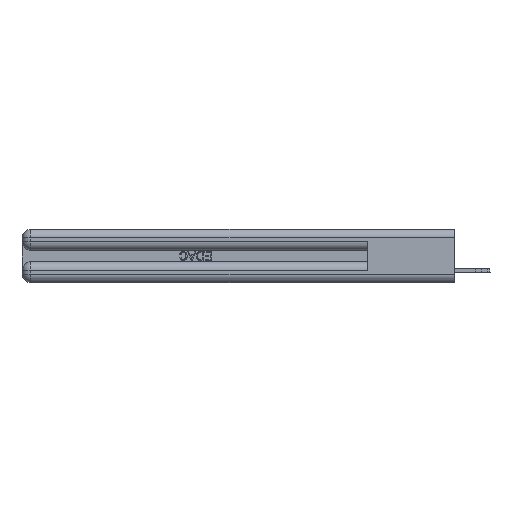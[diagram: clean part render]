
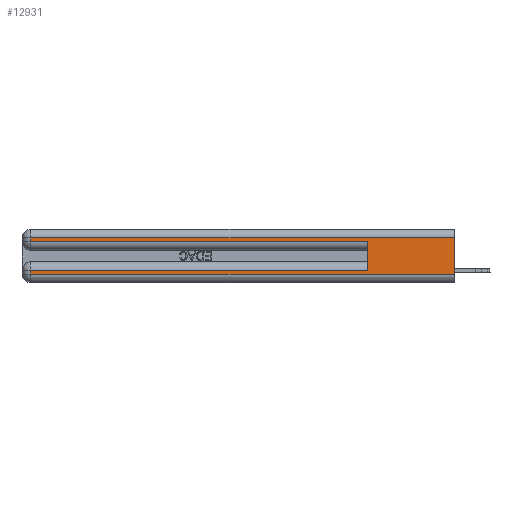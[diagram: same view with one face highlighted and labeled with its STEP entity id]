
A CAD part, left-side view. The second image highlights one B-rep face of the part: STEP entity #12931.
In plain terms, the highlighted planar face has unit normal (-1, 0, 0).
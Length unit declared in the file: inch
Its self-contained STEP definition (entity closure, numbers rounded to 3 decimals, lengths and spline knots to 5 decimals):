
#27 = EDGE_LOOP ( 'NONE', ( #20840, #12368, #30266, #17095, #7942, #33751, #11199, #32306 ) ) ;
#104 = LINE ( 'NONE', #30512, #34752 ) ;
#208 = EDGE_CURVE ( 'NONE', #19348, #15938, #38544, .T. ) ;
#327 = VERTEX_POINT ( 'NONE', #32156 ) ;
#4027 = CARTESIAN_POINT ( 'NONE',  ( 0., 0., 0.06 ) ) ;
#4560 = VERTEX_POINT ( 'NONE', #32407 ) ;
#6367 = DIRECTION ( 'NONE',  ( 0., 1., 0. ) ) ;
#6589 = LINE ( 'NONE', #11337, #21766 ) ;
#6918 = DIRECTION ( 'NONE',  ( 0., -1., 0. ) ) ;
#7942 = ORIENTED_EDGE ( 'NONE', *, *, #22465, .F. ) ;
#8157 = LINE ( 'NONE', #22508, #27714 ) ;
#8779 = CARTESIAN_POINT ( 'NONE',  ( 0., 0.6, 0.285 ) ) ;
#10611 = CARTESIAN_POINT ( 'NONE',  ( 0., 2.94, 0.37 ) ) ;
#10621 = CARTESIAN_POINT ( 'NONE',  ( 0., 2.94, 0.285 ) ) ;
#11097 = CARTESIAN_POINT ( 'NONE',  ( 0., 2.94, 0.31 ) ) ;
#11199 = ORIENTED_EDGE ( 'NONE', *, *, #13962, .T. ) ;
#11329 = CARTESIAN_POINT ( 'NONE',  ( 0., 0., 0.37 ) ) ;
#11337 = CARTESIAN_POINT ( 'NONE',  ( 0., 0., 0.06 ) ) ;
#11460 = DIRECTION ( 'NONE',  ( 1., 0., 0. ) ) ;
#12236 = VECTOR ( 'NONE', #14869, 39.37008 ) ;
#12368 = ORIENTED_EDGE ( 'NONE', *, *, #38593, .T. ) ;
#12931 = ADVANCED_FACE ( 'NONE', ( #22344 ), #33391, .F. ) ;
#13962 = EDGE_CURVE ( 'NONE', #4560, #327, #27676, .T. ) ;
#14600 = LINE ( 'NONE', #20571, #38479 ) ;
#14724 = DIRECTION ( 'NONE',  ( 0., 0., -1. ) ) ;
#14869 = DIRECTION ( 'NONE',  ( 0., 0., -1. ) ) ;
#15903 = CARTESIAN_POINT ( 'NONE',  ( 0., 0., 0.31 ) ) ;
#15938 = VERTEX_POINT ( 'NONE', #4027 ) ;
#17095 = ORIENTED_EDGE ( 'NONE', *, *, #18173, .T. ) ;
#17554 = VERTEX_POINT ( 'NONE', #19187 ) ;
#17614 = DIRECTION ( 'NONE',  ( 0., -1., 0. ) ) ;
#18053 = EDGE_CURVE ( 'NONE', #17554, #4560, #104, .T. ) ;
#18173 = EDGE_CURVE ( 'NONE', #27788, #25254, #39672, .T. ) ;
#19187 = CARTESIAN_POINT ( 'NONE',  ( 0., 0.6, 0.085 ) ) ;
#19348 = VERTEX_POINT ( 'NONE', #34386 ) ;
#19372 = DIRECTION ( 'NONE',  ( 0., 0., -1. ) ) ;
#20571 = CARTESIAN_POINT ( 'NONE',  ( 0., 2.94, 0.37 ) ) ;
#20840 = ORIENTED_EDGE ( 'NONE', *, *, #208, .F. ) ;
#21028 = CARTESIAN_POINT ( 'NONE',  ( 0., 0., 0.37 ) ) ;
#21766 = VECTOR ( 'NONE', #17614, 39.37008 ) ;
#22094 = VECTOR ( 'NONE', #6918, 39.37008 ) ;
#22344 = FACE_OUTER_BOUND ( 'NONE', #27, .T. ) ;
#22465 = EDGE_CURVE ( 'NONE', #17554, #25254, #8157, .T. ) ;
#22508 = CARTESIAN_POINT ( 'NONE',  ( 0., 0.6, 0.145 ) ) ;
#25254 = VERTEX_POINT ( 'NONE', #8779 ) ;
#26817 = DIRECTION ( 'NONE',  ( 0., 0., -1. ) ) ;
#27676 = LINE ( 'NONE', #10611, #36945 ) ;
#27714 = VECTOR ( 'NONE', #32048, 39.37008 ) ;
#27788 = VERTEX_POINT ( 'NONE', #10621 ) ;
#28051 = VECTOR ( 'NONE', #6367, 39.37008 ) ;
#28634 = CARTESIAN_POINT ( 'NONE',  ( 0., 0., 0.285 ) ) ;
#28971 = VERTEX_POINT ( 'NONE', #11097 ) ;
#29470 = EDGE_CURVE ( 'NONE', #327, #15938, #6589, .T. ) ;
#30266 = ORIENTED_EDGE ( 'NONE', *, *, #33594, .T. ) ;
#30512 = CARTESIAN_POINT ( 'NONE',  ( 0., 0., 0.085 ) ) ;
#32048 = DIRECTION ( 'NONE',  ( 0., 0., 1. ) ) ;
#32156 = CARTESIAN_POINT ( 'NONE',  ( 0., 2.94, 0.06 ) ) ;
#32306 = ORIENTED_EDGE ( 'NONE', *, *, #29470, .T. ) ;
#32407 = CARTESIAN_POINT ( 'NONE',  ( 0., 2.94, 0.085 ) ) ;
#33391 = PLANE ( 'NONE',  #35042 ) ;
#33594 = EDGE_CURVE ( 'NONE', #28971, #27788, #14600, .T. ) ;
#33751 = ORIENTED_EDGE ( 'NONE', *, *, #18053, .T. ) ;
#34386 = CARTESIAN_POINT ( 'NONE',  ( 0., 0., 0.31 ) ) ;
#34752 = VECTOR ( 'NONE', #37782, 39.37008 ) ;
#35042 = AXIS2_PLACEMENT_3D ( 'NONE', #11329, #11460, #14724 ) ;
#36357 = LINE ( 'NONE', #15903, #28051 ) ;
#36945 = VECTOR ( 'NONE', #19372, 39.37008 ) ;
#37782 = DIRECTION ( 'NONE',  ( 0., 1., 0. ) ) ;
#38479 = VECTOR ( 'NONE', #26817, 39.37008 ) ;
#38544 = LINE ( 'NONE', #21028, #12236 ) ;
#38593 = EDGE_CURVE ( 'NONE', #19348, #28971, #36357, .T. ) ;
#39672 = LINE ( 'NONE', #28634, #22094 ) ;
